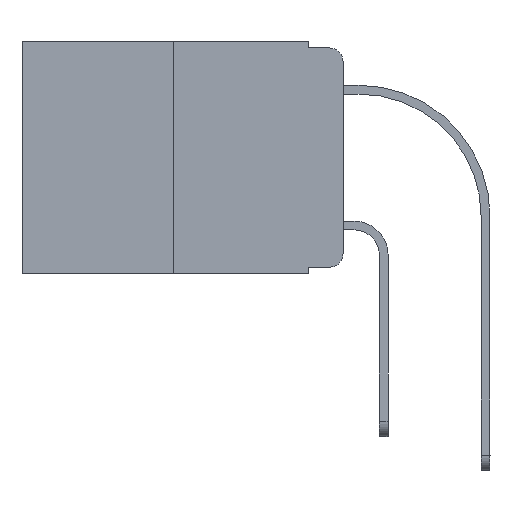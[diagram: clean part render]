
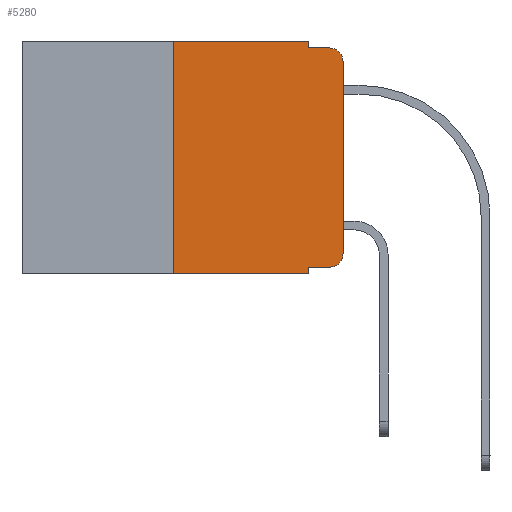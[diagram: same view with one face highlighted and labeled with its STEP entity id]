
A CAD part, left-side view. The second image highlights one B-rep face of the part: STEP entity #5280.
In plain terms, the highlighted planar face has unit normal (-1, 0, 0).
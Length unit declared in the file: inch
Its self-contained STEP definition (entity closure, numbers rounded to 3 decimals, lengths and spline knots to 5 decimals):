
#92 = DIRECTION ( 'NONE',  ( 0., 0., -1. ) ) ;
#131 = DIRECTION ( 'NONE',  ( 0., -1., 0. ) ) ;
#153 = DIRECTION ( 'NONE',  ( -1., 0., 0. ) ) ;
#282 = LINE ( 'NONE', #23331, #25204 ) ;
#604 = CARTESIAN_POINT ( 'NONE',  ( 0., 0.473, 0. ) ) ;
#767 = ORIENTED_EDGE ( 'NONE', *, *, #8443, .T. ) ;
#878 = ORIENTED_EDGE ( 'NONE', *, *, #9826, .F. ) ;
#1774 = CARTESIAN_POINT ( 'NONE',  ( 0., 0.051, 0. ) ) ;
#2148 = ORIENTED_EDGE ( 'NONE', *, *, #24692, .F. ) ;
#2223 = DIRECTION ( 'NONE',  ( 0., 0., 1. ) ) ;
#2513 = VECTOR ( 'NONE', #92, 39.37008 ) ;
#2597 = CARTESIAN_POINT ( 'NONE',  ( 0., 0.051, 0. ) ) ;
#2692 = LINE ( 'NONE', #5356, #23145 ) ;
#3097 = CARTESIAN_POINT ( 'NONE',  ( 0., 0.25, 0. ) ) ;
#3118 = LINE ( 'NONE', #604, #14144 ) ;
#3643 = CIRCLE ( 'NONE', #26111, 0.02 ) ;
#4657 = ORIENTED_EDGE ( 'NONE', *, *, #26582, .F. ) ;
#5280 = ADVANCED_FACE ( 'NONE', ( #19121 ), #6176, .F. ) ;
#5356 = CARTESIAN_POINT ( 'NONE',  ( 0., 0.051, -0.01 ) ) ;
#5750 = ORIENTED_EDGE ( 'NONE', *, *, #20963, .F. ) ;
#6120 = CARTESIAN_POINT ( 'NONE',  ( 0., 0., -0.03 ) ) ;
#6176 = PLANE ( 'NONE',  #18493 ) ;
#6377 = LINE ( 'NONE', #17123, #10930 ) ;
#6881 = CARTESIAN_POINT ( 'NONE',  ( 0., 0.25, -0.343 ) ) ;
#6920 = DIRECTION ( 'NONE',  ( 0., -1., 0. ) ) ;
#7177 = DIRECTION ( 'NONE',  ( 0., 0., -1. ) ) ;
#7530 = CARTESIAN_POINT ( 'NONE',  ( 0., 0.02, -0.01 ) ) ;
#7620 = VERTEX_POINT ( 'NONE', #26506 ) ;
#7689 = LINE ( 'NONE', #22897, #20025 ) ;
#7781 = CIRCLE ( 'NONE', #23509, 0.02 ) ;
#7922 = DIRECTION ( 'NONE',  ( 0., 0., -1. ) ) ;
#8443 = EDGE_CURVE ( 'NONE', #10873, #23832, #7781, .T. ) ;
#8714 = CARTESIAN_POINT ( 'NONE',  ( 0., 0.02, -0.333 ) ) ;
#9785 = EDGE_CURVE ( 'NONE', #7620, #23832, #2692, .T. ) ;
#9826 = EDGE_CURVE ( 'NONE', #16015, #11612, #3118, .T. ) ;
#10044 = VERTEX_POINT ( 'NONE', #12103 ) ;
#10366 = DIRECTION ( 'NONE',  ( 1., 0., 0. ) ) ;
#10528 = EDGE_CURVE ( 'NONE', #14062, #10873, #282, .T. ) ;
#10873 = VERTEX_POINT ( 'NONE', #6120 ) ;
#10930 = VECTOR ( 'NONE', #131, 39.37008 ) ;
#11021 = ORIENTED_EDGE ( 'NONE', *, *, #23336, .T. ) ;
#11190 = EDGE_CURVE ( 'NONE', #13849, #14062, #3643, .T. ) ;
#11612 = VERTEX_POINT ( 'NONE', #2597 ) ;
#11855 = VECTOR ( 'NONE', #22762, 39.37008 ) ;
#12103 = CARTESIAN_POINT ( 'NONE',  ( 0., 0.051, -0.333 ) ) ;
#12619 = DIRECTION ( 'NONE',  ( 0., 0., -1. ) ) ;
#12632 = ORIENTED_EDGE ( 'NONE', *, *, #21965, .T. ) ;
#13811 = CARTESIAN_POINT ( 'NONE',  ( 0., 0.02, -0.03 ) ) ;
#13826 = VERTEX_POINT ( 'NONE', #6881 ) ;
#13849 = VERTEX_POINT ( 'NONE', #8714 ) ;
#14051 = CARTESIAN_POINT ( 'NONE',  ( 0., 0., -0.313 ) ) ;
#14062 = VERTEX_POINT ( 'NONE', #14051 ) ;
#14144 = VECTOR ( 'NONE', #22531, 39.37008 ) ;
#14706 = VECTOR ( 'NONE', #7922, 39.37008 ) ;
#15204 = EDGE_LOOP ( 'NONE', ( #20092, #767, #20826, #5750, #878, #2148, #12632, #4657, #11021, #20546 ) ) ;
#15391 = VERTEX_POINT ( 'NONE', #17400 ) ;
#16015 = VERTEX_POINT ( 'NONE', #3097 ) ;
#16635 = LINE ( 'NONE', #18624, #14706 ) ;
#17123 = CARTESIAN_POINT ( 'NONE',  ( 0., 0.473, -0.343 ) ) ;
#17400 = CARTESIAN_POINT ( 'NONE',  ( 0., 0.051, -0.343 ) ) ;
#18118 = CARTESIAN_POINT ( 'NONE',  ( 0., 0.051, -0.333 ) ) ;
#18493 = AXIS2_PLACEMENT_3D ( 'NONE', #21386, #10366, #12619 ) ;
#18624 = CARTESIAN_POINT ( 'NONE',  ( 0., 0.051, 0. ) ) ;
#19121 = FACE_OUTER_BOUND ( 'NONE', #15204, .T. ) ;
#20025 = VECTOR ( 'NONE', #20800, 39.37008 ) ;
#20092 = ORIENTED_EDGE ( 'NONE', *, *, #10528, .T. ) ;
#20546 = ORIENTED_EDGE ( 'NONE', *, *, #11190, .T. ) ;
#20800 = DIRECTION ( 'NONE',  ( 0., 0., 1. ) ) ;
#20826 = ORIENTED_EDGE ( 'NONE', *, *, #9785, .F. ) ;
#20963 = EDGE_CURVE ( 'NONE', #11612, #7620, #16635, .T. ) ;
#21386 = CARTESIAN_POINT ( 'NONE',  ( 0., 0.473, 0. ) ) ;
#21965 = EDGE_CURVE ( 'NONE', #13826, #15391, #6377, .T. ) ;
#22038 = DIRECTION ( 'NONE',  ( 0., 0., -1. ) ) ;
#22353 = LINE ( 'NONE', #18118, #11855 ) ;
#22531 = DIRECTION ( 'NONE',  ( 0., -1., 0. ) ) ;
#22762 = DIRECTION ( 'NONE',  ( 0., -1., 0. ) ) ;
#22897 = CARTESIAN_POINT ( 'NONE',  ( 0., 0.25, 0. ) ) ;
#23145 = VECTOR ( 'NONE', #6920, 39.37008 ) ;
#23331 = CARTESIAN_POINT ( 'NONE',  ( 0., 0., 0. ) ) ;
#23336 = EDGE_CURVE ( 'NONE', #10044, #13849, #22353, .T. ) ;
#23345 = CARTESIAN_POINT ( 'NONE',  ( 0., 0.02, -0.313 ) ) ;
#23424 = LINE ( 'NONE', #1774, #2513 ) ;
#23509 = AXIS2_PLACEMENT_3D ( 'NONE', #13811, #24507, #7177 ) ;
#23832 = VERTEX_POINT ( 'NONE', #7530 ) ;
#24507 = DIRECTION ( 'NONE',  ( -1., 0., 0. ) ) ;
#24692 = EDGE_CURVE ( 'NONE', #13826, #16015, #7689, .T. ) ;
#25204 = VECTOR ( 'NONE', #2223, 39.37008 ) ;
#26111 = AXIS2_PLACEMENT_3D ( 'NONE', #23345, #153, #22038 ) ;
#26506 = CARTESIAN_POINT ( 'NONE',  ( 0., 0.051, -0.01 ) ) ;
#26582 = EDGE_CURVE ( 'NONE', #10044, #15391, #23424, .T. ) ;
